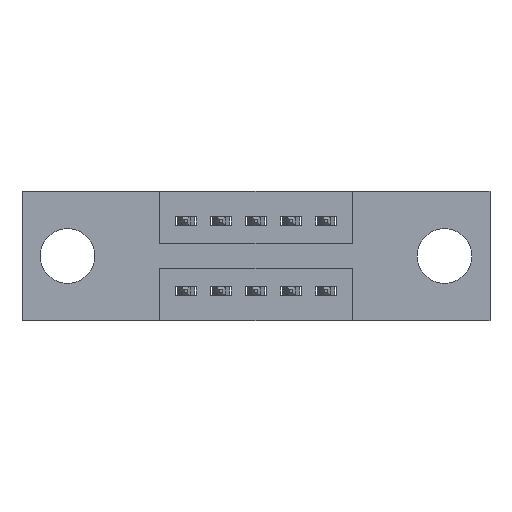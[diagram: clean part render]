
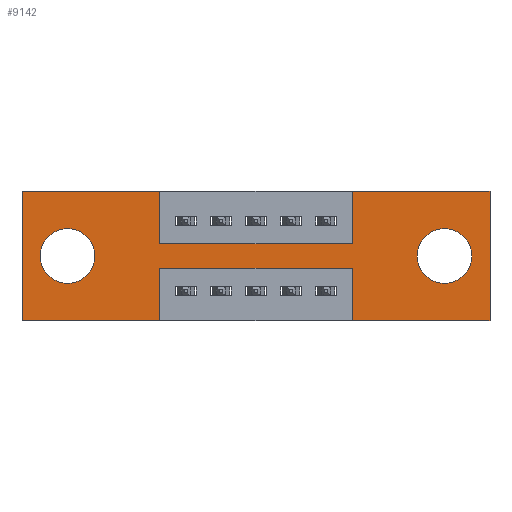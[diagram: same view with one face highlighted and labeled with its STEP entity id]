
A CAD part, front view. The second image highlights one B-rep face of the part: STEP entity #9142.
In plain terms, the highlighted planar face has unit normal (0, -1, 0).
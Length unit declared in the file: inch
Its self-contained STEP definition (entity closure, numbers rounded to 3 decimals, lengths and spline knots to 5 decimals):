
#27 = VERTEX_POINT ( 'NONE', #7105 ) ;
#111 = VECTOR ( 'NONE', #2542, 39.37008 ) ;
#131 = ORIENTED_EDGE ( 'NONE', *, *, #6289, .F. ) ;
#170 = PLANE ( 'NONE',  #5154 ) ;
#179 = VERTEX_POINT ( 'NONE', #672 ) ;
#294 = EDGE_CURVE ( 'NONE', #7900, #7763, #4563, .T. ) ;
#467 = DIRECTION ( 'NONE',  ( 0., 0., 1. ) ) ;
#530 = CARTESIAN_POINT ( 'NONE',  ( 0.9425, 0., -0.22 ) ) ;
#596 = VERTEX_POINT ( 'NONE', #9279 ) ;
#664 = CARTESIAN_POINT ( 'NONE',  ( 0., 0., -0.37 ) ) ;
#672 = CARTESIAN_POINT ( 'NONE',  ( 1.335, 0., -0.37 ) ) ;
#751 = LINE ( 'NONE', #8806, #5881 ) ;
#752 = DIRECTION ( 'NONE',  ( 0., 0., 1. ) ) ;
#778 = VECTOR ( 'NONE', #8770, 39.37008 ) ;
#789 = AXIS2_PLACEMENT_3D ( 'NONE', #1760, #8199, #1903 ) ;
#831 = DIRECTION ( 'NONE',  ( 0., 1., 0. ) ) ;
#846 = ORIENTED_EDGE ( 'NONE', *, *, #3066, .F. ) ;
#1025 = DIRECTION ( 'NONE',  ( -1., 0., 0. ) ) ;
#1051 = CARTESIAN_POINT ( 'NONE',  ( 0.3925, 0., 0. ) ) ;
#1114 = EDGE_CURVE ( 'NONE', #5868, #4108, #7215, .T. ) ;
#1260 = ORIENTED_EDGE ( 'NONE', *, *, #294, .F. ) ;
#1293 = DIRECTION ( 'NONE',  ( -1., 0., 0. ) ) ;
#1313 = ORIENTED_EDGE ( 'NONE', *, *, #5660, .F. ) ;
#1337 = LINE ( 'NONE', #4143, #5867 ) ;
#1602 = EDGE_CURVE ( 'NONE', #6535, #7460, #7483, .T. ) ;
#1617 = DIRECTION ( 'NONE',  ( 1., 0., 0. ) ) ;
#1618 = LINE ( 'NONE', #2952, #778 ) ;
#1639 = VECTOR ( 'NONE', #1293, 39.37008 ) ;
#1702 = LINE ( 'NONE', #1798, #8407 ) ;
#1760 = CARTESIAN_POINT ( 'NONE',  ( 1.205, 0., -0.185 ) ) ;
#1798 = CARTESIAN_POINT ( 'NONE',  ( 0.9425, 0., -0.37 ) ) ;
#1880 = CARTESIAN_POINT ( 'NONE',  ( 0.9425, 0., -0.37 ) ) ;
#1890 = CARTESIAN_POINT ( 'NONE',  ( 1.205, 0., -0.263 ) ) ;
#1903 = DIRECTION ( 'NONE',  ( 0., 0., -1. ) ) ;
#1906 = VECTOR ( 'NONE', #1617, 39.37008 ) ;
#1971 = ORIENTED_EDGE ( 'NONE', *, *, #2425, .F. ) ;
#2009 = EDGE_CURVE ( 'NONE', #7173, #5837, #1702, .T. ) ;
#2093 = CARTESIAN_POINT ( 'NONE',  ( 1.205, 0., -0.185 ) ) ;
#2095 = AXIS2_PLACEMENT_3D ( 'NONE', #5984, #831, #6607 ) ;
#2176 = CARTESIAN_POINT ( 'NONE',  ( 0., 0., 0. ) ) ;
#2182 = VECTOR ( 'NONE', #8291, 39.37008 ) ;
#2321 = DIRECTION ( 'NONE',  ( 1., 0., 0. ) ) ;
#2352 = VERTEX_POINT ( 'NONE', #2176 ) ;
#2357 = LINE ( 'NONE', #5957, #2565 ) ;
#2425 = EDGE_CURVE ( 'NONE', #5837, #27, #4631, .T. ) ;
#2535 = ORIENTED_EDGE ( 'NONE', *, *, #5216, .F. ) ;
#2542 = DIRECTION ( 'NONE',  ( 0., 0., -1. ) ) ;
#2565 = VECTOR ( 'NONE', #752, 39.37008 ) ;
#2709 = DIRECTION ( 'NONE',  ( 0., 0., 1. ) ) ;
#2924 = CARTESIAN_POINT ( 'NONE',  ( 0.13, 0., -0.185 ) ) ;
#2952 = CARTESIAN_POINT ( 'NONE',  ( 0.3925, 0., -0.37 ) ) ;
#3012 = EDGE_CURVE ( 'NONE', #596, #2352, #1337, .T. ) ;
#3066 = EDGE_CURVE ( 'NONE', #179, #7173, #4888, .T. ) ;
#3084 = EDGE_CURVE ( 'NONE', #9163, #6516, #6926, .T. ) ;
#3100 = CARTESIAN_POINT ( 'NONE',  ( 0.3925, 0., -0.15 ) ) ;
#3372 = ORIENTED_EDGE ( 'NONE', *, *, #8279, .F. ) ;
#3458 = DIRECTION ( 'NONE',  ( -1., 0., 0. ) ) ;
#3533 = EDGE_CURVE ( 'NONE', #7763, #179, #6900, .T. ) ;
#3576 = ORIENTED_EDGE ( 'NONE', *, *, #6427, .F. ) ;
#3577 = CARTESIAN_POINT ( 'NONE',  ( 1.335, 0., 0. ) ) ;
#3701 = VERTEX_POINT ( 'NONE', #5708 ) ;
#3769 = FACE_BOUND ( 'NONE', #4343, .T. ) ;
#3818 = DIRECTION ( 'NONE',  ( 0., -1., 0. ) ) ;
#3857 = CARTESIAN_POINT ( 'NONE',  ( 0., 0., 0. ) ) ;
#3872 = CARTESIAN_POINT ( 'NONE',  ( 0.3925, 0., -0.22 ) ) ;
#3941 = CARTESIAN_POINT ( 'NONE',  ( 0.3925, 0., -0.37 ) ) ;
#4067 = AXIS2_PLACEMENT_3D ( 'NONE', #2093, #4282, #7148 ) ;
#4085 = VECTOR ( 'NONE', #3458, 39.37008 ) ;
#4108 = VERTEX_POINT ( 'NONE', #7159 ) ;
#4143 = CARTESIAN_POINT ( 'NONE',  ( 0., 0., 0. ) ) ;
#4146 = CARTESIAN_POINT ( 'NONE',  ( 0.13, 0., -0.263 ) ) ;
#4261 = ORIENTED_EDGE ( 'NONE', *, *, #9101, .T. ) ;
#4282 = DIRECTION ( 'NONE',  ( 0., 1., 0. ) ) ;
#4343 = EDGE_LOOP ( 'NONE', ( #8256, #7152 ) ) ;
#4412 = ORIENTED_EDGE ( 'NONE', *, *, #2009, .F. ) ;
#4563 = LINE ( 'NONE', #6057, #1906 ) ;
#4631 = LINE ( 'NONE', #3872, #8797 ) ;
#4888 = LINE ( 'NONE', #664, #1639 ) ;
#5144 = EDGE_LOOP ( 'NONE', ( #4261, #6086 ) ) ;
#5154 = AXIS2_PLACEMENT_3D ( 'NONE', #8165, #3818, #5368 ) ;
#5179 = CIRCLE ( 'NONE', #9238, 0.078 ) ;
#5216 = EDGE_CURVE ( 'NONE', #7460, #3701, #751, .T. ) ;
#5272 = LINE ( 'NONE', #3857, #6488 ) ;
#5368 = DIRECTION ( 'NONE',  ( 0., 0., -1. ) ) ;
#5475 = CIRCLE ( 'NONE', #789, 0.078 ) ;
#5624 = DIRECTION ( 'NONE',  ( 0., 1., 0. ) ) ;
#5660 = EDGE_CURVE ( 'NONE', #2352, #6535, #5272, .T. ) ;
#5708 = CARTESIAN_POINT ( 'NONE',  ( 0.9425, 0., -0.15 ) ) ;
#5837 = VERTEX_POINT ( 'NONE', #530 ) ;
#5867 = VECTOR ( 'NONE', #2709, 39.37008 ) ;
#5868 = VERTEX_POINT ( 'NONE', #4146 ) ;
#5881 = VECTOR ( 'NONE', #2321, 39.37008 ) ;
#5957 = CARTESIAN_POINT ( 'NONE',  ( 0.9425, 0., 0. ) ) ;
#5984 = CARTESIAN_POINT ( 'NONE',  ( 0.13, 0., -0.185 ) ) ;
#6057 = CARTESIAN_POINT ( 'NONE',  ( 0., 0., 0. ) ) ;
#6086 = ORIENTED_EDGE ( 'NONE', *, *, #1114, .T. ) ;
#6289 = EDGE_CURVE ( 'NONE', #8492, #596, #8615, .T. ) ;
#6427 = EDGE_CURVE ( 'NONE', #3701, #7900, #2357, .T. ) ;
#6488 = VECTOR ( 'NONE', #8160, 39.37008 ) ;
#6516 = VERTEX_POINT ( 'NONE', #1890 ) ;
#6535 = VERTEX_POINT ( 'NONE', #8895 ) ;
#6607 = DIRECTION ( 'NONE',  ( 0., 0., 1. ) ) ;
#6715 = DIRECTION ( 'NONE',  ( 0., 0., 1. ) ) ;
#6900 = LINE ( 'NONE', #9126, #111 ) ;
#6926 = CIRCLE ( 'NONE', #4067, 0.078 ) ;
#7046 = CARTESIAN_POINT ( 'NONE',  ( 0., 0., -0.37 ) ) ;
#7105 = CARTESIAN_POINT ( 'NONE',  ( 0.3925, 0., -0.22 ) ) ;
#7148 = DIRECTION ( 'NONE',  ( 0., 0., -1. ) ) ;
#7152 = ORIENTED_EDGE ( 'NONE', *, *, #8413, .T. ) ;
#7159 = CARTESIAN_POINT ( 'NONE',  ( 0.13, 0., -0.107 ) ) ;
#7173 = VERTEX_POINT ( 'NONE', #1880 ) ;
#7215 = CIRCLE ( 'NONE', #2095, 0.078 ) ;
#7356 = CARTESIAN_POINT ( 'NONE',  ( 0.9425, 0., 0. ) ) ;
#7403 = CARTESIAN_POINT ( 'NONE',  ( 1.205, 0., -0.107 ) ) ;
#7460 = VERTEX_POINT ( 'NONE', #3100 ) ;
#7483 = LINE ( 'NONE', #1051, #2182 ) ;
#7763 = VERTEX_POINT ( 'NONE', #3577 ) ;
#7792 = ORIENTED_EDGE ( 'NONE', *, *, #3012, .F. ) ;
#7900 = VERTEX_POINT ( 'NONE', #7356 ) ;
#8092 = EDGE_LOOP ( 'NONE', ( #3372, #1971, #4412, #846, #8099, #1260, #3576, #2535, #9062, #1313, #7792, #131 ) ) ;
#8099 = ORIENTED_EDGE ( 'NONE', *, *, #3533, .F. ) ;
#8115 = FACE_OUTER_BOUND ( 'NONE', #8092, .T. ) ;
#8160 = DIRECTION ( 'NONE',  ( 1., 0., 0. ) ) ;
#8165 = CARTESIAN_POINT ( 'NONE',  ( 0., 0., -0.37 ) ) ;
#8199 = DIRECTION ( 'NONE',  ( 0., 1., 0. ) ) ;
#8254 = FACE_BOUND ( 'NONE', #5144, .T. ) ;
#8256 = ORIENTED_EDGE ( 'NONE', *, *, #3084, .T. ) ;
#8279 = EDGE_CURVE ( 'NONE', #27, #8492, #1618, .T. ) ;
#8291 = DIRECTION ( 'NONE',  ( 0., 0., -1. ) ) ;
#8407 = VECTOR ( 'NONE', #6715, 39.37008 ) ;
#8413 = EDGE_CURVE ( 'NONE', #6516, #9163, #5475, .T. ) ;
#8492 = VERTEX_POINT ( 'NONE', #3941 ) ;
#8615 = LINE ( 'NONE', #7046, #4085 ) ;
#8770 = DIRECTION ( 'NONE',  ( 0., 0., -1. ) ) ;
#8797 = VECTOR ( 'NONE', #1025, 39.37008 ) ;
#8806 = CARTESIAN_POINT ( 'NONE',  ( 0.3925, 0., -0.15 ) ) ;
#8895 = CARTESIAN_POINT ( 'NONE',  ( 0.3925, 0., 0. ) ) ;
#9062 = ORIENTED_EDGE ( 'NONE', *, *, #1602, .F. ) ;
#9101 = EDGE_CURVE ( 'NONE', #4108, #5868, #5179, .T. ) ;
#9126 = CARTESIAN_POINT ( 'NONE',  ( 1.335, 0., 0. ) ) ;
#9142 = ADVANCED_FACE ( 'NONE', ( #3769, #8254, #8115 ), #170, .T. ) ;
#9163 = VERTEX_POINT ( 'NONE', #7403 ) ;
#9238 = AXIS2_PLACEMENT_3D ( 'NONE', #2924, #5624, #467 ) ;
#9279 = CARTESIAN_POINT ( 'NONE',  ( 0., 0., -0.37 ) ) ;
